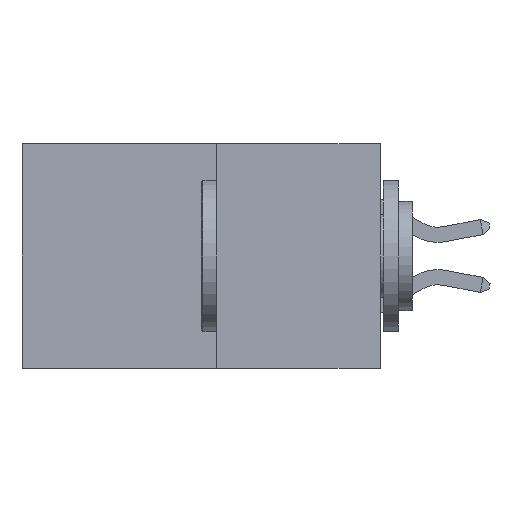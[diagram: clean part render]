
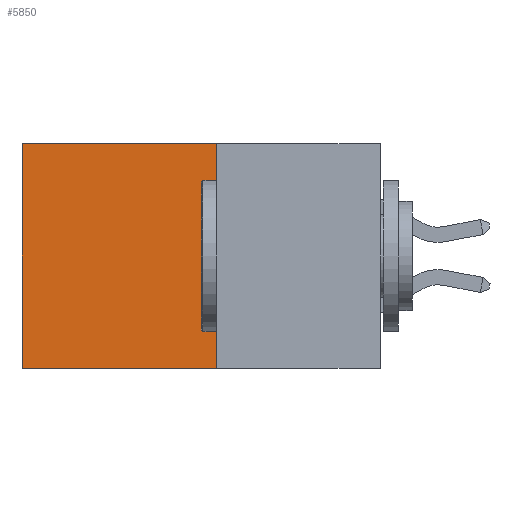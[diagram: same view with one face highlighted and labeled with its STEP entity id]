
A CAD part, left-side view. The second image highlights one B-rep face of the part: STEP entity #5850.
In plain terms, the highlighted planar face has unit normal (-1, 0, 0).
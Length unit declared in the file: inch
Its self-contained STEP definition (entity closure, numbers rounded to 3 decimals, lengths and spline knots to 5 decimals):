
#107 = DIRECTION ( 'NONE',  ( 0., 0., -1. ) ) ;
#919 = VECTOR ( 'NONE', #107, 39.37008 ) ;
#1001 = CARTESIAN_POINT ( 'NONE',  ( 0.277, 0.27, -0.37 ) ) ;
#1257 = VERTEX_POINT ( 'NONE', #7444 ) ;
#1328 = DIRECTION ( 'NONE',  ( 0., 1., 0. ) ) ;
#1463 = FACE_OUTER_BOUND ( 'NONE', #11372, .T. ) ;
#1506 = EDGE_CURVE ( 'NONE', #1257, #1953, #4352, .T. ) ;
#1953 = VERTEX_POINT ( 'NONE', #10016 ) ;
#1980 = ORIENTED_EDGE ( 'NONE', *, *, #8770, .F. ) ;
#2252 = VERTEX_POINT ( 'NONE', #2837 ) ;
#2498 = EDGE_CURVE ( 'NONE', #2252, #1257, #5888, .T. ) ;
#2722 = EDGE_CURVE ( 'NONE', #2252, #6116, #10633, .T. ) ;
#2837 = CARTESIAN_POINT ( 'NONE',  ( 0.277, 0.27, 0. ) ) ;
#2910 = CARTESIAN_POINT ( 'NONE',  ( 0.277, 0.27, -0.37 ) ) ;
#3221 = CARTESIAN_POINT ( 'NONE',  ( 0.277, 0.27, 0. ) ) ;
#3238 = DIRECTION ( 'NONE',  ( 0., 0., -1. ) ) ;
#4084 = VECTOR ( 'NONE', #7354, 39.37008 ) ;
#4352 = LINE ( 'NONE', #10708, #8943 ) ;
#4450 = ORIENTED_EDGE ( 'NONE', *, *, #2498, .T. ) ;
#5340 = DIRECTION ( 'NONE',  ( 0., 0., -1. ) ) ;
#5367 = DIRECTION ( 'NONE',  ( 1., 0., 0. ) ) ;
#5409 = PLANE ( 'NONE',  #10367 ) ;
#5637 = LINE ( 'NONE', #1001, #4084 ) ;
#5850 = ADVANCED_FACE ( 'NONE', ( #1463 ), #5409, .F. ) ;
#5888 = LINE ( 'NONE', #3221, #8072 ) ;
#6116 = VERTEX_POINT ( 'NONE', #2910 ) ;
#6342 = ORIENTED_EDGE ( 'NONE', *, *, #2722, .F. ) ;
#7331 = CARTESIAN_POINT ( 'NONE',  ( 0.277, 0.27, -0.37 ) ) ;
#7354 = DIRECTION ( 'NONE',  ( 0., 1., 0. ) ) ;
#7444 = CARTESIAN_POINT ( 'NONE',  ( 0.277, 0.59, 0. ) ) ;
#8072 = VECTOR ( 'NONE', #1328, 39.37008 ) ;
#8770 = EDGE_CURVE ( 'NONE', #6116, #1953, #5637, .T. ) ;
#8943 = VECTOR ( 'NONE', #3238, 39.37008 ) ;
#9163 = ORIENTED_EDGE ( 'NONE', *, *, #1506, .T. ) ;
#10016 = CARTESIAN_POINT ( 'NONE',  ( 0.277, 0.59, -0.37 ) ) ;
#10367 = AXIS2_PLACEMENT_3D ( 'NONE', #7331, #5367, #5340 ) ;
#10633 = LINE ( 'NONE', #11706, #919 ) ;
#10708 = CARTESIAN_POINT ( 'NONE',  ( 0.277, 0.59, -0.37 ) ) ;
#11372 = EDGE_LOOP ( 'NONE', ( #9163, #1980, #6342, #4450 ) ) ;
#11706 = CARTESIAN_POINT ( 'NONE',  ( 0.277, 0.27, -0.37 ) ) ;
